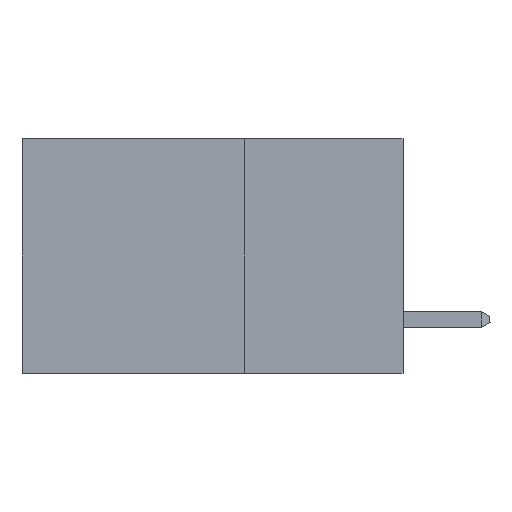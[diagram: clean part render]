
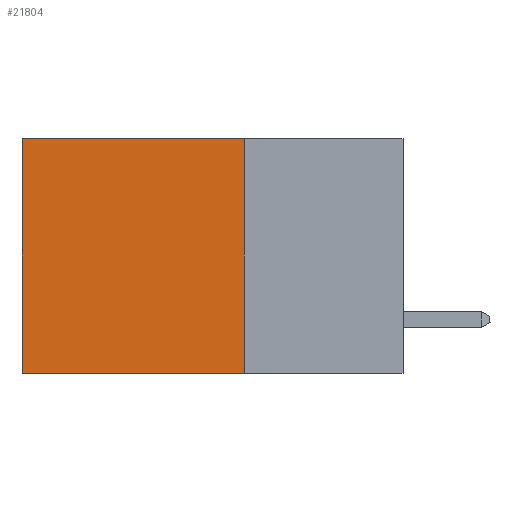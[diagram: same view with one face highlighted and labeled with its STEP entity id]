
A CAD part, left-side view. The second image highlights one B-rep face of the part: STEP entity #21804.
In plain terms, the highlighted planar face has unit normal (-1, 0, 0).
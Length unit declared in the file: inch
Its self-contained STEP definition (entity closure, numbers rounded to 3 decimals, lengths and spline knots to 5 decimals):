
#306 = ORIENTED_EDGE ( 'NONE', *, *, #10688, .F. ) ;
#955 = LINE ( 'NONE', #8129, #13278 ) ;
#1954 = FACE_OUTER_BOUND ( 'NONE', #19769, .T. ) ;
#2609 = VERTEX_POINT ( 'NONE', #13172 ) ;
#4486 = VECTOR ( 'NONE', #21338, 39.37008 ) ;
#5059 = AXIS2_PLACEMENT_3D ( 'NONE', #20059, #19463, #23696 ) ;
#5700 = CARTESIAN_POINT ( 'NONE',  ( 0.2875, 0.6, 0. ) ) ;
#6172 = VECTOR ( 'NONE', #11788, 39.37008 ) ;
#7283 = LINE ( 'NONE', #13925, #19853 ) ;
#7486 = EDGE_CURVE ( 'NONE', #19411, #12801, #955, .T. ) ;
#8129 = CARTESIAN_POINT ( 'NONE',  ( 0.2875, 0.25, 0. ) ) ;
#8803 = CARTESIAN_POINT ( 'NONE',  ( 0.2875, 0.25, -0.37 ) ) ;
#9225 = ORIENTED_EDGE ( 'NONE', *, *, #7486, .T. ) ;
#10688 = EDGE_CURVE ( 'NONE', #2609, #19135, #23865, .T. ) ;
#11788 = DIRECTION ( 'NONE',  ( 0., 1., 0. ) ) ;
#12279 = CARTESIAN_POINT ( 'NONE',  ( 0.2875, 0.25, 0. ) ) ;
#12801 = VERTEX_POINT ( 'NONE', #5700 ) ;
#13172 = CARTESIAN_POINT ( 'NONE',  ( 0.2875, 0.25, -0.37 ) ) ;
#13278 = VECTOR ( 'NONE', #23758, 39.37008 ) ;
#13333 = ORIENTED_EDGE ( 'NONE', *, *, #23604, .T. ) ;
#13925 = CARTESIAN_POINT ( 'NONE',  ( 0.2875, 0.6, 0. ) ) ;
#14569 = EDGE_CURVE ( 'NONE', #19411, #2609, #18923, .T. ) ;
#14913 = ORIENTED_EDGE ( 'NONE', *, *, #14569, .F. ) ;
#14972 = CARTESIAN_POINT ( 'NONE',  ( 0.2875, 0.6, -0.37 ) ) ;
#18923 = LINE ( 'NONE', #24688, #4486 ) ;
#19135 = VERTEX_POINT ( 'NONE', #14972 ) ;
#19411 = VERTEX_POINT ( 'NONE', #12279 ) ;
#19463 = DIRECTION ( 'NONE',  ( 1., 0., 0. ) ) ;
#19769 = EDGE_LOOP ( 'NONE', ( #13333, #306, #14913, #9225 ) ) ;
#19853 = VECTOR ( 'NONE', #21722, 39.37008 ) ;
#20059 = CARTESIAN_POINT ( 'NONE',  ( 0.2875, 0.25, 0. ) ) ;
#21338 = DIRECTION ( 'NONE',  ( 0., 0., -1. ) ) ;
#21722 = DIRECTION ( 'NONE',  ( 0., 0., -1. ) ) ;
#21759 = PLANE ( 'NONE',  #5059 ) ;
#21804 = ADVANCED_FACE ( 'NONE', ( #1954 ), #21759, .F. ) ;
#23604 = EDGE_CURVE ( 'NONE', #12801, #19135, #7283, .T. ) ;
#23696 = DIRECTION ( 'NONE',  ( 0., 0., -1. ) ) ;
#23758 = DIRECTION ( 'NONE',  ( 0., 1., 0. ) ) ;
#23865 = LINE ( 'NONE', #8803, #6172 ) ;
#24688 = CARTESIAN_POINT ( 'NONE',  ( 0.2875, 0.25, 0. ) ) ;
